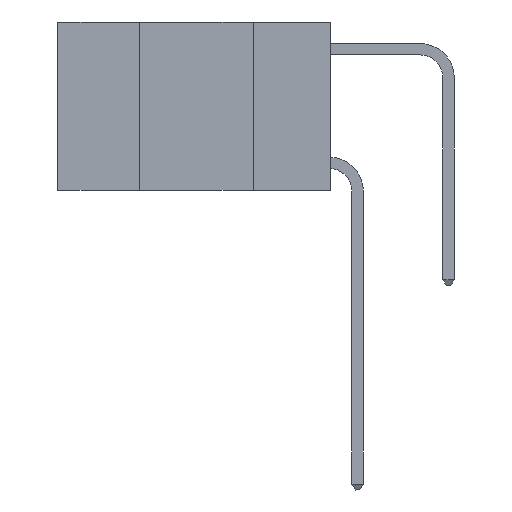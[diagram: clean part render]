
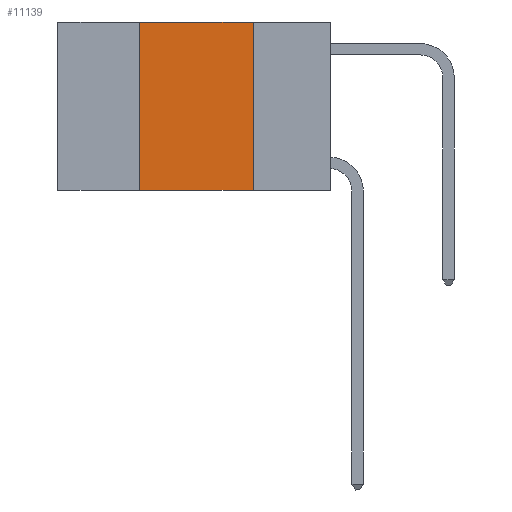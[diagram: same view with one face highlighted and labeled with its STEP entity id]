
A CAD part, left-side view. The second image highlights one B-rep face of the part: STEP entity #11139.
In plain terms, the highlighted planar face has unit normal (-1, 0, 0).
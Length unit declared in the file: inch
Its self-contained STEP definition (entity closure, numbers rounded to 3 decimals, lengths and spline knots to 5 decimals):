
#132 = AXIS2_PLACEMENT_3D ( 'NONE', #7096, #1355, #6970 ) ;
#488 = VECTOR ( 'NONE', #5895, 39.37008 ) ;
#1036 = EDGE_CURVE ( 'NONE', #1172, #2944, #2323, .T. ) ;
#1172 = VERTEX_POINT ( 'NONE', #10146 ) ;
#1355 = DIRECTION ( 'NONE',  ( 1., 0., 0. ) ) ;
#1533 = EDGE_CURVE ( 'NONE', #4206, #1172, #7842, .T. ) ;
#1647 = ORIENTED_EDGE ( 'NONE', *, *, #1036, .F. ) ;
#2139 = DIRECTION ( 'NONE',  ( 0., 0., -1. ) ) ;
#2186 = VECTOR ( 'NONE', #2139, 39.37008 ) ;
#2323 = LINE ( 'NONE', #11711, #2186 ) ;
#2745 = EDGE_CURVE ( 'NONE', #10357, #4206, #5759, .T. ) ;
#2944 = VERTEX_POINT ( 'NONE', #8715 ) ;
#3017 = VECTOR ( 'NONE', #7330, 39.37008 ) ;
#3224 = PLANE ( 'NONE',  #132 ) ;
#3350 = FACE_OUTER_BOUND ( 'NONE', #9843, .T. ) ;
#3550 = CARTESIAN_POINT ( 'NONE',  ( 0., 0.42, 0. ) ) ;
#4206 = VERTEX_POINT ( 'NONE', #3550 ) ;
#4859 = CARTESIAN_POINT ( 'NONE',  ( 0., 0.42, 0. ) ) ;
#5135 = DIRECTION ( 'NONE',  ( 0., -1., 0. ) ) ;
#5747 = ORIENTED_EDGE ( 'NONE', *, *, #1533, .F. ) ;
#5759 = LINE ( 'NONE', #4859, #488 ) ;
#5895 = DIRECTION ( 'NONE',  ( 0., 0., 1. ) ) ;
#6970 = DIRECTION ( 'NONE',  ( 0., 0., -1. ) ) ;
#7096 = CARTESIAN_POINT ( 'NONE',  ( 0., 0.6, 0. ) ) ;
#7330 = DIRECTION ( 'NONE',  ( 0., -1., 0. ) ) ;
#7333 = CARTESIAN_POINT ( 'NONE',  ( 0., 0.42, -0.37 ) ) ;
#7771 = ORIENTED_EDGE ( 'NONE', *, *, #2745, .F. ) ;
#7842 = LINE ( 'NONE', #10059, #3017 ) ;
#8715 = CARTESIAN_POINT ( 'NONE',  ( 0., 0.17, -0.37 ) ) ;
#9843 = EDGE_LOOP ( 'NONE', ( #1647, #5747, #7771, #10177 ) ) ;
#10059 = CARTESIAN_POINT ( 'NONE',  ( 0., 0.6, 0. ) ) ;
#10146 = CARTESIAN_POINT ( 'NONE',  ( 0., 0.17, 0. ) ) ;
#10177 = ORIENTED_EDGE ( 'NONE', *, *, #11167, .T. ) ;
#10357 = VERTEX_POINT ( 'NONE', #7333 ) ;
#10719 = LINE ( 'NONE', #11808, #11730 ) ;
#11139 = ADVANCED_FACE ( 'NONE', ( #3350 ), #3224, .F. ) ;
#11167 = EDGE_CURVE ( 'NONE', #10357, #2944, #10719, .T. ) ;
#11711 = CARTESIAN_POINT ( 'NONE',  ( 0., 0.17, 0. ) ) ;
#11730 = VECTOR ( 'NONE', #5135, 39.37008 ) ;
#11808 = CARTESIAN_POINT ( 'NONE',  ( 0., 0.6, -0.37 ) ) ;
